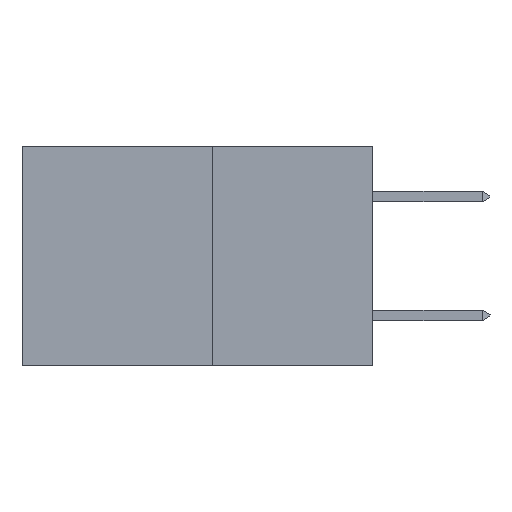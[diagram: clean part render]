
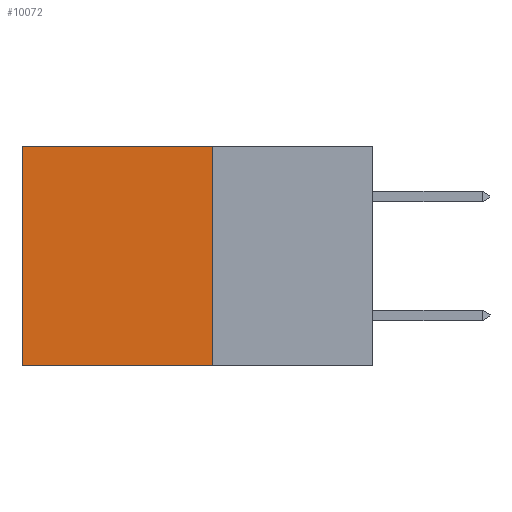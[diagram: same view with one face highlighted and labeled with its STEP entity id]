
A CAD part, left-side view. The second image highlights one B-rep face of the part: STEP entity #10072.
In plain terms, the highlighted planar face has unit normal (-1, 0, 0).
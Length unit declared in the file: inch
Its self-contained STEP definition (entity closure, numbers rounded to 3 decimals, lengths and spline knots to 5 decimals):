
#1522 = VECTOR ( 'NONE', #28287, 39.37008 ) ;
#1946 = LINE ( 'NONE', #6404, #29037 ) ;
#2336 = LINE ( 'NONE', #17701, #1522 ) ;
#3692 = PLANE ( 'NONE',  #24746 ) ;
#3977 = VERTEX_POINT ( 'NONE', #17646 ) ;
#5561 = ORIENTED_EDGE ( 'NONE', *, *, #15405, .T. ) ;
#6352 = DIRECTION ( 'NONE',  ( 1., 0., 0. ) ) ;
#6404 = CARTESIAN_POINT ( 'NONE',  ( 0.277, 0.27, -0.37 ) ) ;
#6783 = VERTEX_POINT ( 'NONE', #15590 ) ;
#8418 = VERTEX_POINT ( 'NONE', #10350 ) ;
#8541 = VECTOR ( 'NONE', #32230, 39.37008 ) ;
#9044 = DIRECTION ( 'NONE',  ( 0., 1., 0. ) ) ;
#9672 = CARTESIAN_POINT ( 'NONE',  ( 0.277, 0.27, -0.37 ) ) ;
#10072 = ADVANCED_FACE ( 'NONE', ( #24697 ), #3692, .F. ) ;
#10350 = CARTESIAN_POINT ( 'NONE',  ( 0.277, 0.59, 0. ) ) ;
#12832 = EDGE_CURVE ( 'NONE', #15098, #3977, #1946, .T. ) ;
#12866 = EDGE_LOOP ( 'NONE', ( #22860, #13684, #29982, #5561 ) ) ;
#13092 = EDGE_CURVE ( 'NONE', #8418, #3977, #2336, .T. ) ;
#13684 = ORIENTED_EDGE ( 'NONE', *, *, #12832, .F. ) ;
#13881 = CARTESIAN_POINT ( 'NONE',  ( 0.277, 0.27, 0. ) ) ;
#15098 = VERTEX_POINT ( 'NONE', #9672 ) ;
#15405 = EDGE_CURVE ( 'NONE', #6783, #8418, #27271, .T. ) ;
#15590 = CARTESIAN_POINT ( 'NONE',  ( 0.277, 0.27, 0. ) ) ;
#17646 = CARTESIAN_POINT ( 'NONE',  ( 0.277, 0.59, -0.37 ) ) ;
#17701 = CARTESIAN_POINT ( 'NONE',  ( 0.277, 0.59, -0.37 ) ) ;
#21984 = CARTESIAN_POINT ( 'NONE',  ( 0.277, 0.27, -0.37 ) ) ;
#22425 = LINE ( 'NONE', #29626, #8541 ) ;
#22860 = ORIENTED_EDGE ( 'NONE', *, *, #13092, .T. ) ;
#24296 = DIRECTION ( 'NONE',  ( 0., 1., 0. ) ) ;
#24671 = DIRECTION ( 'NONE',  ( 0., 0., -1. ) ) ;
#24697 = FACE_OUTER_BOUND ( 'NONE', #12866, .T. ) ;
#24746 = AXIS2_PLACEMENT_3D ( 'NONE', #21984, #6352, #24671 ) ;
#27271 = LINE ( 'NONE', #13881, #33369 ) ;
#28287 = DIRECTION ( 'NONE',  ( 0., 0., -1. ) ) ;
#29037 = VECTOR ( 'NONE', #9044, 39.37008 ) ;
#29626 = CARTESIAN_POINT ( 'NONE',  ( 0.277, 0.27, -0.37 ) ) ;
#29982 = ORIENTED_EDGE ( 'NONE', *, *, #30757, .F. ) ;
#30757 = EDGE_CURVE ( 'NONE', #6783, #15098, #22425, .T. ) ;
#32230 = DIRECTION ( 'NONE',  ( 0., 0., -1. ) ) ;
#33369 = VECTOR ( 'NONE', #24296, 39.37008 ) ;
